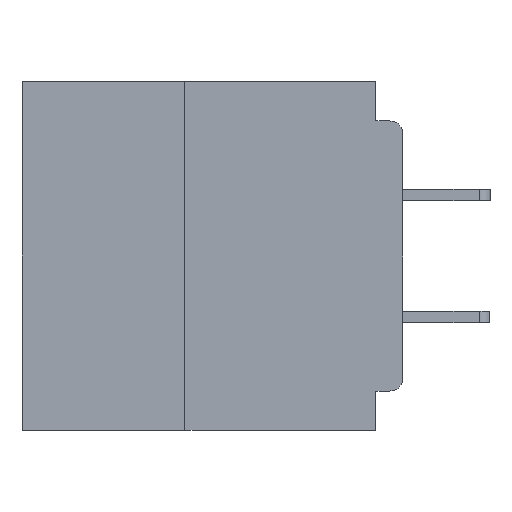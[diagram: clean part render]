
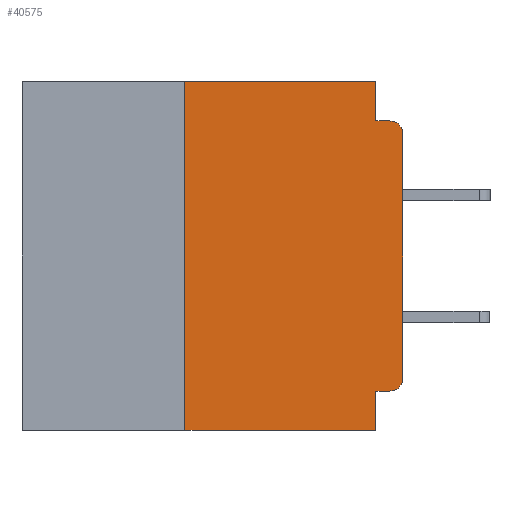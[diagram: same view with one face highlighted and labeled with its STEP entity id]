
A CAD part, left-side view. The second image highlights one B-rep face of the part: STEP entity #40575.
In plain terms, the highlighted planar face has unit normal (-1, 0, 0).
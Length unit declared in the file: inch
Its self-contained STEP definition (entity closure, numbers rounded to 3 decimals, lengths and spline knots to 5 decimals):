
#398 = VECTOR ( 'NONE', #36355, 39.37008 ) ;
#547 = CIRCLE ( 'NONE', #10876, 0.015 ) ;
#1008 = DIRECTION ( 'NONE',  ( 1., 0., 0. ) ) ;
#1224 = VERTEX_POINT ( 'NONE', #29474 ) ;
#1817 = VERTEX_POINT ( 'NONE', #15938 ) ;
#1948 = FACE_OUTER_BOUND ( 'NONE', #44029, .T. ) ;
#3142 = LINE ( 'NONE', #14460, #398 ) ;
#3374 = CARTESIAN_POINT ( 'NONE',  ( 0., 0.031, 0. ) ) ;
#4645 = DIRECTION ( 'NONE',  ( 0., 0., 1. ) ) ;
#4815 = AXIS2_PLACEMENT_3D ( 'NONE', #18463, #1008, #31513 ) ;
#5124 = VECTOR ( 'NONE', #30868, 39.37008 ) ;
#5547 = VECTOR ( 'NONE', #21019, 39.37008 ) ;
#9474 = ORIENTED_EDGE ( 'NONE', *, *, #36748, .F. ) ;
#9693 = CARTESIAN_POINT ( 'NONE',  ( 0., 0.031, -0.4 ) ) ;
#10019 = ORIENTED_EDGE ( 'NONE', *, *, #18281, .F. ) ;
#10274 = VECTOR ( 'NONE', #15256, 39.37008 ) ;
#10876 = AXIS2_PLACEMENT_3D ( 'NONE', #43166, #17100, #47507 ) ;
#12052 = CARTESIAN_POINT ( 'NONE',  ( 0., 0., -0.34 ) ) ;
#12479 = CARTESIAN_POINT ( 'NONE',  ( 0., 0.25, -0.4 ) ) ;
#14460 = CARTESIAN_POINT ( 'NONE',  ( 0., 0., -0.355 ) ) ;
#15256 = DIRECTION ( 'NONE',  ( 0., -1., 0. ) ) ;
#15938 = CARTESIAN_POINT ( 'NONE',  ( 0., 0.015, -0.355 ) ) ;
#16766 = LINE ( 'NONE', #43822, #5124 ) ;
#17100 = DIRECTION ( 'NONE',  ( -1., 0., 0. ) ) ;
#17484 = VERTEX_POINT ( 'NONE', #12052 ) ;
#18281 = EDGE_CURVE ( 'NONE', #39677, #18615, #46939, .T. ) ;
#18463 = CARTESIAN_POINT ( 'NONE',  ( 0., 0.437, 0. ) ) ;
#18571 = VERTEX_POINT ( 'NONE', #23712 ) ;
#18615 = VERTEX_POINT ( 'NONE', #41607 ) ;
#18713 = ORIENTED_EDGE ( 'NONE', *, *, #46322, .T. ) ;
#19238 = VECTOR ( 'NONE', #32904, 39.37008 ) ;
#19740 = VERTEX_POINT ( 'NONE', #49975 ) ;
#20130 = EDGE_CURVE ( 'NONE', #1817, #17484, #33418, .T. ) ;
#21019 = DIRECTION ( 'NONE',  ( 0., 0., -1. ) ) ;
#22020 = DIRECTION ( 'NONE',  ( 0., 0., -1. ) ) ;
#22107 = EDGE_CURVE ( 'NONE', #1817, #1224, #3142, .T. ) ;
#22248 = CARTESIAN_POINT ( 'NONE',  ( 0., 0.015, -0.34 ) ) ;
#23712 = CARTESIAN_POINT ( 'NONE',  ( 0., 0., -0.06 ) ) ;
#26631 = DIRECTION ( 'NONE',  ( 0., 0., -1. ) ) ;
#28294 = LINE ( 'NONE', #52321, #48704 ) ;
#28479 = EDGE_CURVE ( 'NONE', #49310, #19740, #53755, .T. ) ;
#28522 = CARTESIAN_POINT ( 'NONE',  ( 0., 0.25, -0.4 ) ) ;
#29474 = CARTESIAN_POINT ( 'NONE',  ( 0., 0.031, -0.355 ) ) ;
#30119 = LINE ( 'NONE', #3374, #5547 ) ;
#30403 = CARTESIAN_POINT ( 'NONE',  ( 0., 0., -0.045 ) ) ;
#30868 = DIRECTION ( 'NONE',  ( 0., -1., 0. ) ) ;
#30954 = ORIENTED_EDGE ( 'NONE', *, *, #34761, .T. ) ;
#31364 = VECTOR ( 'NONE', #4645, 39.37008 ) ;
#31513 = DIRECTION ( 'NONE',  ( 0., 0., -1. ) ) ;
#32488 = ORIENTED_EDGE ( 'NONE', *, *, #45481, .F. ) ;
#32558 = CARTESIAN_POINT ( 'NONE',  ( 0., 0.437, -0.4 ) ) ;
#32904 = DIRECTION ( 'NONE',  ( 0., 0., 1. ) ) ;
#33418 = CIRCLE ( 'NONE', #40998, 0.015 ) ;
#33503 = ORIENTED_EDGE ( 'NONE', *, *, #37416, .F. ) ;
#34079 = EDGE_CURVE ( 'NONE', #49310, #44050, #44979, .T. ) ;
#34761 = EDGE_CURVE ( 'NONE', #18571, #18615, #547, .T. ) ;
#34797 = DIRECTION ( 'NONE',  ( 0., -1., 0. ) ) ;
#34988 = CARTESIAN_POINT ( 'NONE',  ( 0., 0., 0. ) ) ;
#36136 = ORIENTED_EDGE ( 'NONE', *, *, #34079, .T. ) ;
#36355 = DIRECTION ( 'NONE',  ( 0., 1., 0. ) ) ;
#36748 = EDGE_CURVE ( 'NONE', #1224, #44050, #28294, .T. ) ;
#37416 = EDGE_CURVE ( 'NONE', #19740, #40832, #16766, .T. ) ;
#39677 = VERTEX_POINT ( 'NONE', #51499 ) ;
#40128 = CARTESIAN_POINT ( 'NONE',  ( 0., 0.031, 0. ) ) ;
#40575 = ADVANCED_FACE ( 'NONE', ( #1948 ), #53082, .F. ) ;
#40832 = VERTEX_POINT ( 'NONE', #40128 ) ;
#40886 = ORIENTED_EDGE ( 'NONE', *, *, #20130, .T. ) ;
#40998 = AXIS2_PLACEMENT_3D ( 'NONE', #22248, #52545, #26631 ) ;
#41607 = CARTESIAN_POINT ( 'NONE',  ( 0., 0.015, -0.045 ) ) ;
#41955 = ORIENTED_EDGE ( 'NONE', *, *, #22107, .F. ) ;
#43166 = CARTESIAN_POINT ( 'NONE',  ( 0., 0.015, -0.06 ) ) ;
#43822 = CARTESIAN_POINT ( 'NONE',  ( 0., 0.437, 0. ) ) ;
#44029 = EDGE_LOOP ( 'NONE', ( #18713, #30954, #10019, #32488, #33503, #48301, #36136, #9474, #41955, #40886 ) ) ;
#44050 = VERTEX_POINT ( 'NONE', #9693 ) ;
#44979 = LINE ( 'NONE', #32558, #10274 ) ;
#45481 = EDGE_CURVE ( 'NONE', #40832, #39677, #30119, .T. ) ;
#46322 = EDGE_CURVE ( 'NONE', #17484, #18571, #54344, .T. ) ;
#46939 = LINE ( 'NONE', #30403, #51912 ) ;
#47507 = DIRECTION ( 'NONE',  ( 0., 0., -1. ) ) ;
#48301 = ORIENTED_EDGE ( 'NONE', *, *, #28479, .F. ) ;
#48704 = VECTOR ( 'NONE', #22020, 39.37008 ) ;
#49310 = VERTEX_POINT ( 'NONE', #12479 ) ;
#49975 = CARTESIAN_POINT ( 'NONE',  ( 0., 0.25, 0. ) ) ;
#51499 = CARTESIAN_POINT ( 'NONE',  ( 0., 0.031, -0.045 ) ) ;
#51912 = VECTOR ( 'NONE', #34797, 39.37008 ) ;
#52321 = CARTESIAN_POINT ( 'NONE',  ( 0., 0.031, -0.4 ) ) ;
#52545 = DIRECTION ( 'NONE',  ( -1., 0., 0. ) ) ;
#53082 = PLANE ( 'NONE',  #4815 ) ;
#53755 = LINE ( 'NONE', #28522, #19238 ) ;
#54344 = LINE ( 'NONE', #34988, #31364 ) ;
